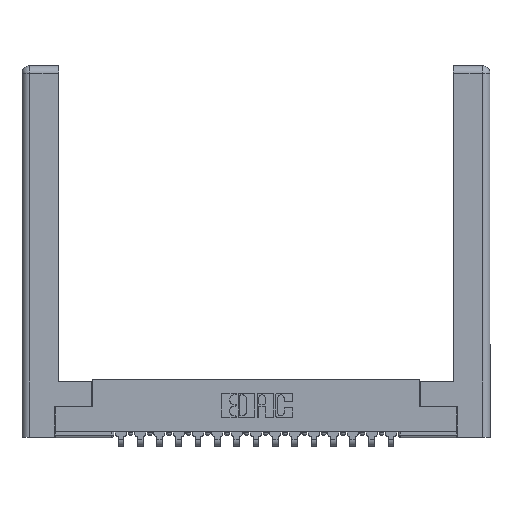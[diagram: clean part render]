
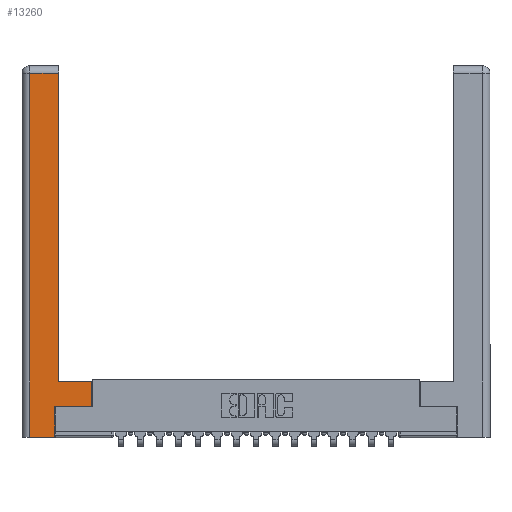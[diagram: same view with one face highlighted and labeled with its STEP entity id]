
A CAD part, top view. The second image highlights one B-rep face of the part: STEP entity #13260.
In plain terms, the highlighted planar face has unit normal (0, 0, 1).
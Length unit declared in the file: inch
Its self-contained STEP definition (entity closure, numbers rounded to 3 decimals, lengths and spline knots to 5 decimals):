
#170 = VERTEX_POINT ( 'NONE', #9934 ) ;
#233 = DIRECTION ( 'NONE',  ( 0., 1., 0. ) ) ;
#361 = ORIENTED_EDGE ( 'NONE', *, *, #3385, .T. ) ;
#654 = DIRECTION ( 'NONE',  ( -1., 0., 0. ) ) ;
#1525 = ORIENTED_EDGE ( 'NONE', *, *, #9547, .T. ) ;
#1577 = EDGE_CURVE ( 'NONE', #8060, #5354, #17515, .T. ) ;
#1586 = DIRECTION ( 'NONE',  ( 0., -1., 0. ) ) ;
#1710 = CARTESIAN_POINT ( 'NONE',  ( 0.295, 0.45, 0. ) ) ;
#1990 = VECTOR ( 'NONE', #9097, 39.37008 ) ;
#1997 = PLANE ( 'NONE',  #8627 ) ;
#2749 = LINE ( 'NONE', #4653, #9909 ) ;
#2933 = CARTESIAN_POINT ( 'NONE',  ( 0.565, 0.245, 0. ) ) ;
#3163 = ORIENTED_EDGE ( 'NONE', *, *, #7660, .T. ) ;
#3385 = EDGE_CURVE ( 'NONE', #12882, #8347, #16262, .T. ) ;
#3501 = VECTOR ( 'NONE', #16793, 39.37008 ) ;
#4090 = VECTOR ( 'NONE', #1586, 39.37008 ) ;
#4216 = CARTESIAN_POINT ( 'NONE',  ( 0.295, 2.94, 0. ) ) ;
#4389 = CARTESIAN_POINT ( 'NONE',  ( 0.295, 0.45, 0. ) ) ;
#4639 = LINE ( 'NONE', #8973, #15646 ) ;
#4653 = CARTESIAN_POINT ( 'NONE',  ( 0.565, 0.45, 0. ) ) ;
#5280 = DIRECTION ( 'NONE',  ( 1., 0., 0. ) ) ;
#5300 = EDGE_CURVE ( 'NONE', #5354, #13503, #6660, .T. ) ;
#5354 = VERTEX_POINT ( 'NONE', #1710 ) ;
#6256 = EDGE_CURVE ( 'NONE', #170, #17830, #17491, .T. ) ;
#6386 = DIRECTION ( 'NONE',  ( -1., 0., 0. ) ) ;
#6660 = LINE ( 'NONE', #12505, #15986 ) ;
#6833 = CARTESIAN_POINT ( 'NONE',  ( 0.0615, 2.94, 0. ) ) ;
#6848 = DIRECTION ( 'NONE',  ( 0., 1., 0. ) ) ;
#7660 = EDGE_CURVE ( 'NONE', #13503, #12882, #4639, .T. ) ;
#7927 = VECTOR ( 'NONE', #5280, 39.37008 ) ;
#8060 = VERTEX_POINT ( 'NONE', #12011 ) ;
#8089 = EDGE_LOOP ( 'NONE', ( #13550, #3163, #361, #14535, #14794, #1525, #10971, #9832 ) ) ;
#8347 = VERTEX_POINT ( 'NONE', #8648 ) ;
#8627 = AXIS2_PLACEMENT_3D ( 'NONE', #15416, #12373, #654 ) ;
#8648 = CARTESIAN_POINT ( 'NONE',  ( 0.0615, 0., 0. ) ) ;
#8973 = CARTESIAN_POINT ( 'NONE',  ( 0.0615, 2.94, 0. ) ) ;
#9097 = DIRECTION ( 'NONE',  ( 1., 0., 0. ) ) ;
#9547 = EDGE_CURVE ( 'NONE', #17830, #12722, #12495, .T. ) ;
#9832 = ORIENTED_EDGE ( 'NONE', *, *, #1577, .T. ) ;
#9909 = VECTOR ( 'NONE', #233, 39.37008 ) ;
#9934 = CARTESIAN_POINT ( 'NONE',  ( 0.265, 0., 0. ) ) ;
#10971 = ORIENTED_EDGE ( 'NONE', *, *, #13954, .T. ) ;
#11572 = CARTESIAN_POINT ( 'NONE',  ( 0.265, 0.245, 0. ) ) ;
#12011 = CARTESIAN_POINT ( 'NONE',  ( 0.565, 0.45, 0. ) ) ;
#12373 = DIRECTION ( 'NONE',  ( 0., 0., -1. ) ) ;
#12495 = LINE ( 'NONE', #18296, #7927 ) ;
#12505 = CARTESIAN_POINT ( 'NONE',  ( 0.295, 3., 0. ) ) ;
#12722 = VERTEX_POINT ( 'NONE', #2933 ) ;
#12882 = VERTEX_POINT ( 'NONE', #6833 ) ;
#13260 = ADVANCED_FACE ( 'NONE', ( #13803 ), #1997, .F. ) ;
#13483 = CARTESIAN_POINT ( 'NONE',  ( 0.0615, 0., 0. ) ) ;
#13503 = VERTEX_POINT ( 'NONE', #4216 ) ;
#13550 = ORIENTED_EDGE ( 'NONE', *, *, #5300, .T. ) ;
#13803 = FACE_OUTER_BOUND ( 'NONE', #8089, .T. ) ;
#13954 = EDGE_CURVE ( 'NONE', #12722, #8060, #2749, .T. ) ;
#14535 = ORIENTED_EDGE ( 'NONE', *, *, #16175, .T. ) ;
#14794 = ORIENTED_EDGE ( 'NONE', *, *, #6256, .T. ) ;
#15414 = CARTESIAN_POINT ( 'NONE',  ( 0.265, 0.245, 0. ) ) ;
#15416 = CARTESIAN_POINT ( 'NONE',  ( 0., 0., 0. ) ) ;
#15646 = VECTOR ( 'NONE', #6386, 39.37008 ) ;
#15986 = VECTOR ( 'NONE', #6848, 39.37008 ) ;
#16151 = DIRECTION ( 'NONE',  ( 0., 1., 0. ) ) ;
#16175 = EDGE_CURVE ( 'NONE', #8347, #170, #16270, .T. ) ;
#16177 = CARTESIAN_POINT ( 'NONE',  ( 0.265, 0., 0. ) ) ;
#16262 = LINE ( 'NONE', #13483, #4090 ) ;
#16270 = LINE ( 'NONE', #16177, #1990 ) ;
#16613 = VECTOR ( 'NONE', #16151, 39.37008 ) ;
#16793 = DIRECTION ( 'NONE',  ( -1., 0., 0. ) ) ;
#17491 = LINE ( 'NONE', #11572, #16613 ) ;
#17515 = LINE ( 'NONE', #4389, #3501 ) ;
#17830 = VERTEX_POINT ( 'NONE', #15414 ) ;
#18296 = CARTESIAN_POINT ( 'NONE',  ( 0.565, 0.245, 0. ) ) ;
